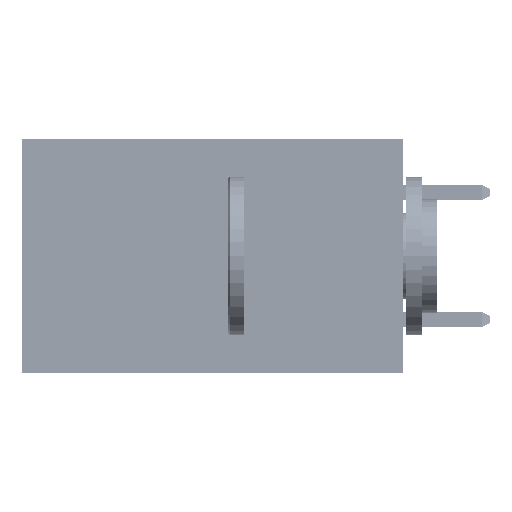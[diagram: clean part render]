
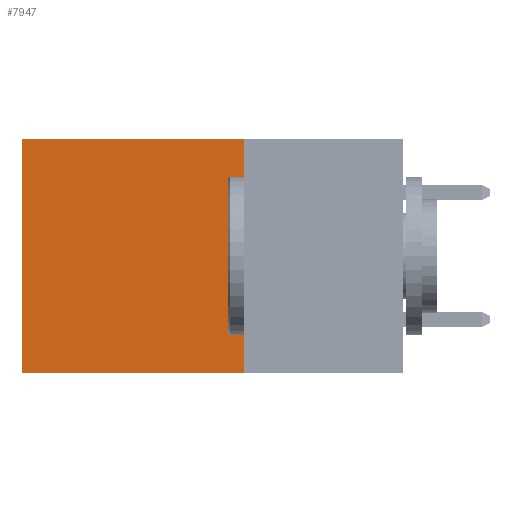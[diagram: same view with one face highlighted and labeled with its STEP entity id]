
A CAD part, left-side view. The second image highlights one B-rep face of the part: STEP entity #7947.
In plain terms, the highlighted planar face has unit normal (-1, 0, 0).
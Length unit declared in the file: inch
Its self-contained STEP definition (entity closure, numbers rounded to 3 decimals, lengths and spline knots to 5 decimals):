
#295 = VECTOR ( 'NONE', #19322, 39.37008 ) ;
#501 = CARTESIAN_POINT ( 'NONE',  ( 0.2875, 0.25, 0. ) ) ;
#930 = CARTESIAN_POINT ( 'NONE',  ( 0.2875, 0.25, -0.37 ) ) ;
#1232 = VECTOR ( 'NONE', #45745, 39.37008 ) ;
#1701 = VECTOR ( 'NONE', #14101, 39.37008 ) ;
#1708 = DIRECTION ( 'NONE',  ( 0., 0., -1. ) ) ;
#2125 = EDGE_LOOP ( 'NONE', ( #30207, #28535, #30699, #36993 ) ) ;
#3840 = VECTOR ( 'NONE', #1708, 39.37008 ) ;
#4289 = EDGE_CURVE ( 'NONE', #30724, #38720, #31693, .T. ) ;
#5569 = PLANE ( 'NONE',  #38633 ) ;
#6259 = EDGE_CURVE ( 'NONE', #30724, #41046, #9392, .T. ) ;
#6966 = CARTESIAN_POINT ( 'NONE',  ( 0.2875, 0.6, 0. ) ) ;
#7947 = ADVANCED_FACE ( 'NONE', ( #13882 ), #5569, .F. ) ;
#7973 = LINE ( 'NONE', #45361, #295 ) ;
#9392 = LINE ( 'NONE', #28666, #1701 ) ;
#9409 = DIRECTION ( 'NONE',  ( 0., 0., -1. ) ) ;
#10952 = LINE ( 'NONE', #38543, #3840 ) ;
#13882 = FACE_OUTER_BOUND ( 'NONE', #2125, .T. ) ;
#14101 = DIRECTION ( 'NONE',  ( 0., 0., -1. ) ) ;
#19322 = DIRECTION ( 'NONE',  ( 0., 1., 0. ) ) ;
#19888 = EDGE_CURVE ( 'NONE', #38720, #31230, #10952, .T. ) ;
#27704 = CARTESIAN_POINT ( 'NONE',  ( 0.2875, 0.25, 0. ) ) ;
#28535 = ORIENTED_EDGE ( 'NONE', *, *, #38146, .F. ) ;
#28666 = CARTESIAN_POINT ( 'NONE',  ( 0.2875, 0.25, 0. ) ) ;
#30207 = ORIENTED_EDGE ( 'NONE', *, *, #19888, .T. ) ;
#30699 = ORIENTED_EDGE ( 'NONE', *, *, #6259, .F. ) ;
#30724 = VERTEX_POINT ( 'NONE', #33128 ) ;
#31230 = VERTEX_POINT ( 'NONE', #31787 ) ;
#31693 = LINE ( 'NONE', #501, #1232 ) ;
#31787 = CARTESIAN_POINT ( 'NONE',  ( 0.2875, 0.6, -0.37 ) ) ;
#33128 = CARTESIAN_POINT ( 'NONE',  ( 0.2875, 0.25, 0. ) ) ;
#35531 = DIRECTION ( 'NONE',  ( 1., 0., 0. ) ) ;
#36993 = ORIENTED_EDGE ( 'NONE', *, *, #4289, .T. ) ;
#38146 = EDGE_CURVE ( 'NONE', #41046, #31230, #7973, .T. ) ;
#38543 = CARTESIAN_POINT ( 'NONE',  ( 0.2875, 0.6, 0. ) ) ;
#38633 = AXIS2_PLACEMENT_3D ( 'NONE', #27704, #35531, #9409 ) ;
#38720 = VERTEX_POINT ( 'NONE', #6966 ) ;
#41046 = VERTEX_POINT ( 'NONE', #930 ) ;
#45361 = CARTESIAN_POINT ( 'NONE',  ( 0.2875, 0.25, -0.37 ) ) ;
#45745 = DIRECTION ( 'NONE',  ( 0., 1., 0. ) ) ;
